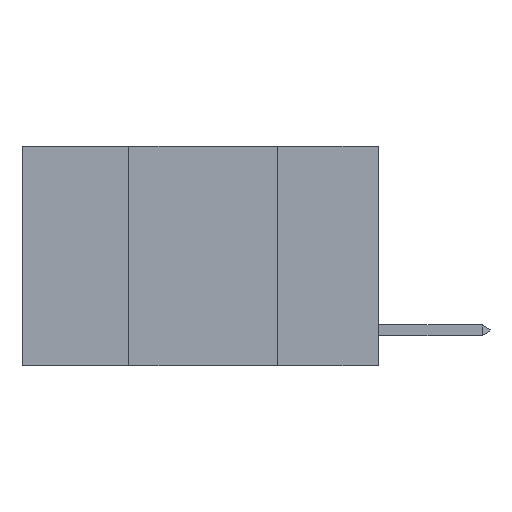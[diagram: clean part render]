
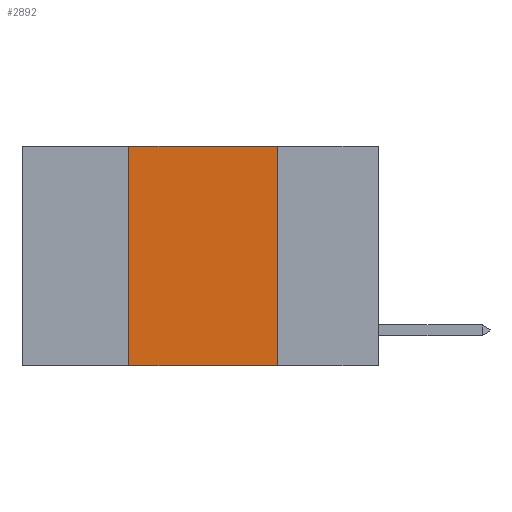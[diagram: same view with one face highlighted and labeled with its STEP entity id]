
A CAD part, left-side view. The second image highlights one B-rep face of the part: STEP entity #2892.
In plain terms, the highlighted planar face has unit normal (-1, 0, 0).
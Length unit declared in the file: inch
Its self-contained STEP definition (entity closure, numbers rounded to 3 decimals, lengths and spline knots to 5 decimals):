
#305 = EDGE_CURVE ( 'NONE', #10221, #1407, #14484, .T. ) ;
#531 = EDGE_CURVE ( 'NONE', #10983, #8129, #5243, .T. ) ;
#1407 = VERTEX_POINT ( 'NONE', #8602 ) ;
#1472 = EDGE_CURVE ( 'NONE', #8129, #10221, #15185, .T. ) ;
#1734 = LINE ( 'NONE', #6278, #8135 ) ;
#1805 = DIRECTION ( 'NONE',  ( 0., 0., 1. ) ) ;
#1850 = ORIENTED_EDGE ( 'NONE', *, *, #14105, .T. ) ;
#2825 = CARTESIAN_POINT ( 'NONE',  ( 0., 0.42, 0. ) ) ;
#2892 = ADVANCED_FACE ( 'NONE', ( #13653 ), #2919, .F. ) ;
#2919 = PLANE ( 'NONE',  #8654 ) ;
#4244 = DIRECTION ( 'NONE',  ( 0., 0., -1. ) ) ;
#4482 = ORIENTED_EDGE ( 'NONE', *, *, #305, .F. ) ;
#4843 = VECTOR ( 'NONE', #1805, 39.37008 ) ;
#5013 = DIRECTION ( 'NONE',  ( 0., -1., 0. ) ) ;
#5243 = LINE ( 'NONE', #12195, #4843 ) ;
#5484 = DIRECTION ( 'NONE',  ( 0., 0., -1. ) ) ;
#6278 = CARTESIAN_POINT ( 'NONE',  ( 0., 0.6, -0.37 ) ) ;
#6490 = CARTESIAN_POINT ( 'NONE',  ( 0., 0.17, 0. ) ) ;
#8103 = CARTESIAN_POINT ( 'NONE',  ( 0., 0.17, 0. ) ) ;
#8129 = VERTEX_POINT ( 'NONE', #2825 ) ;
#8135 = VECTOR ( 'NONE', #5013, 39.37008 ) ;
#8602 = CARTESIAN_POINT ( 'NONE',  ( 0., 0.17, -0.37 ) ) ;
#8654 = AXIS2_PLACEMENT_3D ( 'NONE', #11678, #12897, #5484 ) ;
#10221 = VERTEX_POINT ( 'NONE', #6490 ) ;
#10983 = VERTEX_POINT ( 'NONE', #15232 ) ;
#11300 = VECTOR ( 'NONE', #4244, 39.37008 ) ;
#11678 = CARTESIAN_POINT ( 'NONE',  ( 0., 0.6, 0. ) ) ;
#11884 = ORIENTED_EDGE ( 'NONE', *, *, #531, .F. ) ;
#11987 = VECTOR ( 'NONE', #14435, 39.37008 ) ;
#12195 = CARTESIAN_POINT ( 'NONE',  ( 0., 0.42, 0. ) ) ;
#12897 = DIRECTION ( 'NONE',  ( 1., 0., 0. ) ) ;
#13653 = FACE_OUTER_BOUND ( 'NONE', #15396, .T. ) ;
#14105 = EDGE_CURVE ( 'NONE', #10983, #1407, #1734, .T. ) ;
#14435 = DIRECTION ( 'NONE',  ( 0., -1., 0. ) ) ;
#14484 = LINE ( 'NONE', #8103, #11300 ) ;
#15081 = ORIENTED_EDGE ( 'NONE', *, *, #1472, .F. ) ;
#15185 = LINE ( 'NONE', #15853, #11987 ) ;
#15232 = CARTESIAN_POINT ( 'NONE',  ( 0., 0.42, -0.37 ) ) ;
#15396 = EDGE_LOOP ( 'NONE', ( #4482, #15081, #11884, #1850 ) ) ;
#15853 = CARTESIAN_POINT ( 'NONE',  ( 0., 0.6, 0. ) ) ;
